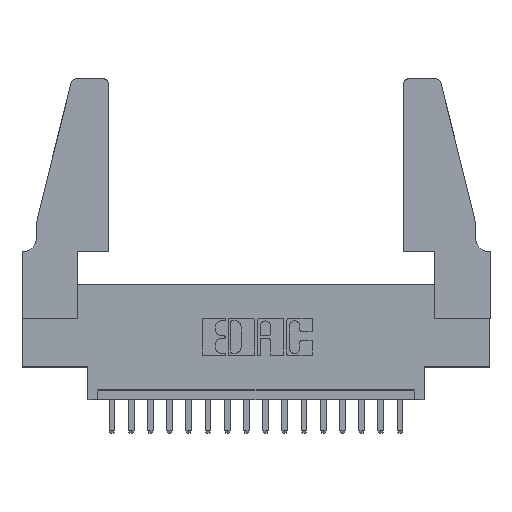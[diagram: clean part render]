
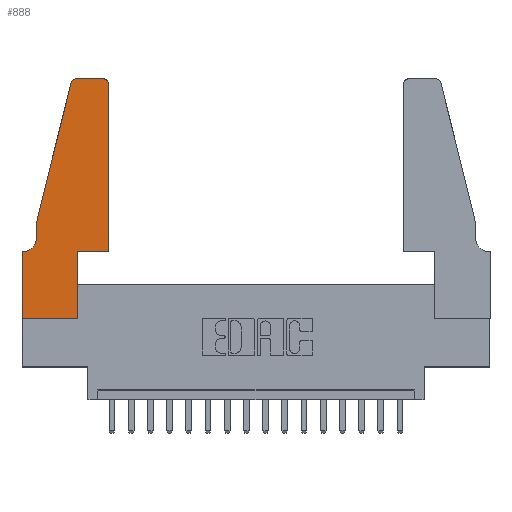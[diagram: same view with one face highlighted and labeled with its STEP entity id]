
A CAD part, top view. The second image highlights one B-rep face of the part: STEP entity #888.
In plain terms, the highlighted planar face has unit normal (0, 0, 1).
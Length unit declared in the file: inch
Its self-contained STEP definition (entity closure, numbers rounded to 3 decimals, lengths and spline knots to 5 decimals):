
#156 = EDGE_CURVE ( 'NONE', #7639, #12595, #16177, .T. ) ;
#444 = LINE ( 'NONE', #8298, #13887 ) ;
#450 = DIRECTION ( 'NONE',  ( 1., 0., 0. ) ) ;
#637 = CARTESIAN_POINT ( 'NONE',  ( 0.0055, 0.42, 0.37 ) ) ;
#833 = CARTESIAN_POINT ( 'NONE',  ( 0., 0., 0.37 ) ) ;
#863 = VERTEX_POINT ( 'NONE', #6613 ) ;
#884 = PLANE ( 'NONE',  #15893 ) ;
#888 = ADVANCED_FACE ( 'NONE', ( #15918 ), #884, .T. ) ;
#1076 = CIRCLE ( 'NONE', #2173, 0.03 ) ;
#1613 = AXIS2_PLACEMENT_3D ( 'NONE', #7331, #12890, #450 ) ;
#1680 = EDGE_LOOP ( 'NONE', ( #15781, #3378, #8954, #6992, #9502, #4776, #4272, #4974, #12007, #9283, #12402, #2919 ) ) ;
#1859 = CARTESIAN_POINT ( 'NONE',  ( 0.4205, 1.25, 0.37 ) ) ;
#2173 = AXIS2_PLACEMENT_3D ( 'NONE', #5717, #5658, #7062 ) ;
#2177 = DIRECTION ( 'NONE',  ( 1., 0., 0. ) ) ;
#2598 = VERTEX_POINT ( 'NONE', #17367 ) ;
#2843 = EDGE_CURVE ( 'NONE', #863, #14941, #3083, .T. ) ;
#2844 = CARTESIAN_POINT ( 'NONE',  ( 0.0755, 0.5, 0.37 ) ) ;
#2919 = ORIENTED_EDGE ( 'NONE', *, *, #13949, .T. ) ;
#3065 = CARTESIAN_POINT ( 'NONE',  ( 0.4505, 0.35, 0.37 ) ) ;
#3083 = LINE ( 'NONE', #2844, #4407 ) ;
#3378 = ORIENTED_EDGE ( 'NONE', *, *, #16137, .T. ) ;
#3541 = CARTESIAN_POINT ( 'NONE',  ( 0.2865, 0.35, 0.37 ) ) ;
#4066 = EDGE_CURVE ( 'NONE', #2598, #863, #5551, .T. ) ;
#4108 = DIRECTION ( 'NONE',  ( 0., -1., 0. ) ) ;
#4272 = ORIENTED_EDGE ( 'NONE', *, *, #5186, .T. ) ;
#4407 = VECTOR ( 'NONE', #4108, 39.37008 ) ;
#4508 = CARTESIAN_POINT ( 'NONE',  ( 0., 0., 0.37 ) ) ;
#4585 = CARTESIAN_POINT ( 'NONE',  ( 0.4505, 0.35, 0.37 ) ) ;
#4680 = DIRECTION ( 'NONE',  ( 0., -1., 0. ) ) ;
#4686 = VERTEX_POINT ( 'NONE', #15153 ) ;
#4776 = ORIENTED_EDGE ( 'NONE', *, *, #9023, .T. ) ;
#4792 = CARTESIAN_POINT ( 'NONE',  ( 0.2605, 1.25, 0.37 ) ) ;
#4974 = ORIENTED_EDGE ( 'NONE', *, *, #7269, .T. ) ;
#5186 = EDGE_CURVE ( 'NONE', #14040, #11060, #12206, .T. ) ;
#5198 = CARTESIAN_POINT ( 'NONE',  ( 0., 0.35, 0.37 ) ) ;
#5441 = AXIS2_PLACEMENT_3D ( 'NONE', #637, #17285, #10333 ) ;
#5522 = VERTEX_POINT ( 'NONE', #12462 ) ;
#5551 = LINE ( 'NONE', #10100, #14619 ) ;
#5658 = DIRECTION ( 'NONE',  ( 0., 0., 1. ) ) ;
#5717 = CARTESIAN_POINT ( 'NONE',  ( 0.4205, 1.22, 0.37 ) ) ;
#6424 = EDGE_CURVE ( 'NONE', #5522, #11957, #444, .T. ) ;
#6554 = DIRECTION ( 'NONE',  ( 0., 0., 1. ) ) ;
#6613 = CARTESIAN_POINT ( 'NONE',  ( 0.0755, 0.5, 0.37 ) ) ;
#6689 = LINE ( 'NONE', #14717, #12301 ) ;
#6992 = ORIENTED_EDGE ( 'NONE', *, *, #2843, .T. ) ;
#7062 = DIRECTION ( 'NONE',  ( 1., 0., 0. ) ) ;
#7237 = DIRECTION ( 'NONE',  ( -0.239, -0.971, 0. ) ) ;
#7269 = EDGE_CURVE ( 'NONE', #11060, #5522, #11479, .T. ) ;
#7331 = CARTESIAN_POINT ( 'NONE',  ( 0.284, 1.22, 0.37 ) ) ;
#7421 = DIRECTION ( 'NONE',  ( 1., 0., 0. ) ) ;
#7575 = VECTOR ( 'NONE', #2177, 39.37008 ) ;
#7639 = VERTEX_POINT ( 'NONE', #4585 ) ;
#7765 = DIRECTION ( 'NONE',  ( -1., 0., 0. ) ) ;
#8298 = CARTESIAN_POINT ( 'NONE',  ( 0.2865, 0.35, 0.37 ) ) ;
#8416 = CARTESIAN_POINT ( 'NONE',  ( 0.0755, 0.42, 0.37 ) ) ;
#8749 = VERTEX_POINT ( 'NONE', #17860 ) ;
#8762 = CARTESIAN_POINT ( 'NONE',  ( 0., 0.35, 0.37 ) ) ;
#8794 = VECTOR ( 'NONE', #7421, 39.37008 ) ;
#8954 = ORIENTED_EDGE ( 'NONE', *, *, #4066, .T. ) ;
#9023 = EDGE_CURVE ( 'NONE', #8749, #14040, #6689, .T. ) ;
#9266 = EDGE_CURVE ( 'NONE', #11957, #7639, #10108, .T. ) ;
#9283 = ORIENTED_EDGE ( 'NONE', *, *, #9266, .T. ) ;
#9502 = ORIENTED_EDGE ( 'NONE', *, *, #13019, .T. ) ;
#10100 = CARTESIAN_POINT ( 'NONE',  ( 0.0755, 0.5, 0.37 ) ) ;
#10108 = LINE ( 'NONE', #10868, #8794 ) ;
#10333 = DIRECTION ( 'NONE',  ( -1., 0., 0. ) ) ;
#10742 = CARTESIAN_POINT ( 'NONE',  ( 0., 0., 0.37 ) ) ;
#10853 = DIRECTION ( 'NONE',  ( 0., 1., 0. ) ) ;
#10868 = CARTESIAN_POINT ( 'NONE',  ( 0.4505, 0.35, 0.37 ) ) ;
#11060 = VERTEX_POINT ( 'NONE', #10742 ) ;
#11479 = LINE ( 'NONE', #833, #7575 ) ;
#11957 = VERTEX_POINT ( 'NONE', #3541 ) ;
#12007 = ORIENTED_EDGE ( 'NONE', *, *, #6424, .T. ) ;
#12206 = LINE ( 'NONE', #4508, #13276 ) ;
#12301 = VECTOR ( 'NONE', #7765, 39.37008 ) ;
#12402 = ORIENTED_EDGE ( 'NONE', *, *, #156, .T. ) ;
#12462 = CARTESIAN_POINT ( 'NONE',  ( 0.2865, 0., 0.37 ) ) ;
#12595 = VERTEX_POINT ( 'NONE', #13692 ) ;
#12890 = DIRECTION ( 'NONE',  ( 0., 0., 1. ) ) ;
#12953 = VECTOR ( 'NONE', #15446, 39.37008 ) ;
#12970 = VERTEX_POINT ( 'NONE', #1859 ) ;
#13019 = EDGE_CURVE ( 'NONE', #14941, #8749, #13897, .T. ) ;
#13276 = VECTOR ( 'NONE', #4680, 39.37008 ) ;
#13324 = DIRECTION ( 'NONE',  ( 1., 0., 0. ) ) ;
#13346 = CIRCLE ( 'NONE', #1613, 0.03 ) ;
#13692 = CARTESIAN_POINT ( 'NONE',  ( 0.4505, 1.22, 0.37 ) ) ;
#13887 = VECTOR ( 'NONE', #10853, 39.37008 ) ;
#13897 = CIRCLE ( 'NONE', #5441, 0.07 ) ;
#13949 = EDGE_CURVE ( 'NONE', #12595, #12970, #1076, .T. ) ;
#14040 = VERTEX_POINT ( 'NONE', #8762 ) ;
#14619 = VECTOR ( 'NONE', #7237, 39.37008 ) ;
#14651 = EDGE_CURVE ( 'NONE', #12970, #4686, #14686, .T. ) ;
#14686 = LINE ( 'NONE', #4792, #16627 ) ;
#14717 = CARTESIAN_POINT ( 'NONE',  ( 0.0755, 0.35, 0.37 ) ) ;
#14941 = VERTEX_POINT ( 'NONE', #8416 ) ;
#15153 = CARTESIAN_POINT ( 'NONE',  ( 0.284, 1.25, 0.37 ) ) ;
#15446 = DIRECTION ( 'NONE',  ( 0., 1., 0. ) ) ;
#15781 = ORIENTED_EDGE ( 'NONE', *, *, #14651, .T. ) ;
#15893 = AXIS2_PLACEMENT_3D ( 'NONE', #5198, #6554, #13324 ) ;
#15918 = FACE_OUTER_BOUND ( 'NONE', #1680, .T. ) ;
#16137 = EDGE_CURVE ( 'NONE', #4686, #2598, #13346, .T. ) ;
#16177 = LINE ( 'NONE', #3065, #12953 ) ;
#16627 = VECTOR ( 'NONE', #16758, 39.37008 ) ;
#16758 = DIRECTION ( 'NONE',  ( -1., 0., 0. ) ) ;
#17285 = DIRECTION ( 'NONE',  ( 0., 0., -1. ) ) ;
#17367 = CARTESIAN_POINT ( 'NONE',  ( 0.25487, 1.22718, 0.37 ) ) ;
#17860 = CARTESIAN_POINT ( 'NONE',  ( 0.0055, 0.35, 0.37 ) ) ;
